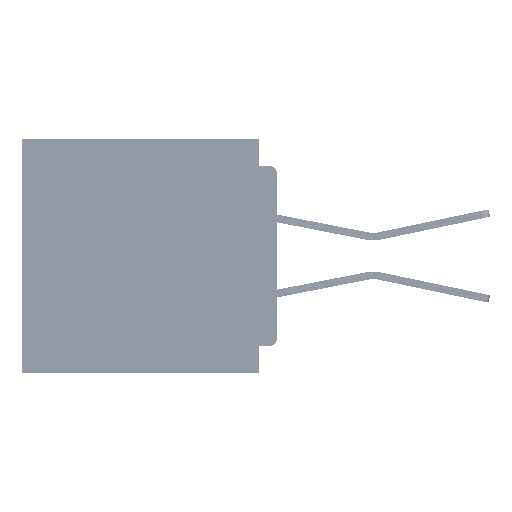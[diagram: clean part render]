
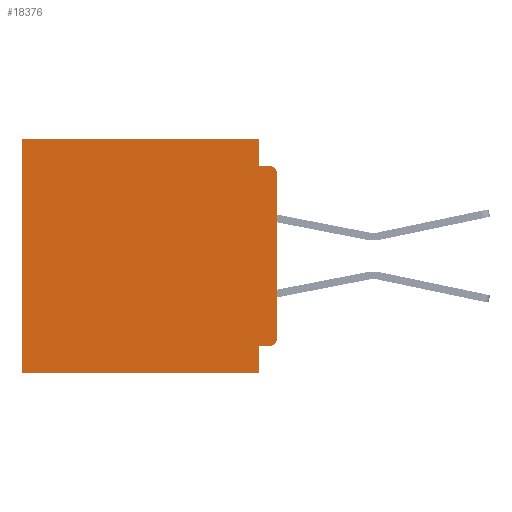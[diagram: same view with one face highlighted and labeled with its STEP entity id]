
A CAD part, left-side view. The second image highlights one B-rep face of the part: STEP entity #18376.
In plain terms, the highlighted planar face has unit normal (-1, 0, 0).
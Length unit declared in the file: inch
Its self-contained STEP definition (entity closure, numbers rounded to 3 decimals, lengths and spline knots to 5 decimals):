
#213 = CARTESIAN_POINT ( 'NONE',  ( 0.3, 0.437, -0.4 ) ) ;
#479 = ORIENTED_EDGE ( 'NONE', *, *, #10741, .F. ) ;
#855 = FACE_OUTER_BOUND ( 'NONE', #14915, .T. ) ;
#1376 = LINE ( 'NONE', #213, #41180 ) ;
#2153 = DIRECTION ( 'NONE',  ( 0., 0., -1. ) ) ;
#3269 = DIRECTION ( 'NONE',  ( 0., 1., 0. ) ) ;
#3931 = LINE ( 'NONE', #19192, #29967 ) ;
#5414 = DIRECTION ( 'NONE',  ( 0., 0., -1. ) ) ;
#5662 = CARTESIAN_POINT ( 'NONE',  ( 0.3, 0.031, -0.045 ) ) ;
#7006 = CARTESIAN_POINT ( 'NONE',  ( 0.3, 0.015, -0.34 ) ) ;
#7553 = VERTEX_POINT ( 'NONE', #53003 ) ;
#8582 = CARTESIAN_POINT ( 'NONE',  ( 0.3, 0., -0.045 ) ) ;
#9204 = LINE ( 'NONE', #8582, #48821 ) ;
#9430 = CARTESIAN_POINT ( 'NONE',  ( 0.3, 0.437, -0.4 ) ) ;
#9541 = VECTOR ( 'NONE', #35898, 39.37008 ) ;
#10218 = CARTESIAN_POINT ( 'NONE',  ( 0.3, 0., -0.4 ) ) ;
#10741 = EDGE_CURVE ( 'NONE', #64204, #25860, #42358, .T. ) ;
#12268 = EDGE_CURVE ( 'NONE', #49437, #56496, #38239, .T. ) ;
#12282 = EDGE_CURVE ( 'NONE', #60415, #41325, #48625, .T. ) ;
#12359 = DIRECTION ( 'NONE',  ( 0., 0., -1. ) ) ;
#13957 = DIRECTION ( 'NONE',  ( 0., -1., 0. ) ) ;
#14915 = EDGE_LOOP ( 'NONE', ( #58551, #46555, #37774, #23265, #29747, #54612, #479, #41886, #33028, #25817 ) ) ;
#17399 = VERTEX_POINT ( 'NONE', #35720 ) ;
#17871 = CARTESIAN_POINT ( 'NONE',  ( 0.3, 0.015, -0.06 ) ) ;
#18376 = ADVANCED_FACE ( 'NONE', ( #855 ), #38282, .F. ) ;
#19192 = CARTESIAN_POINT ( 'NONE',  ( 0.3, 0., 0. ) ) ;
#20373 = EDGE_CURVE ( 'NONE', #17399, #25860, #1376, .T. ) ;
#22192 = CARTESIAN_POINT ( 'NONE',  ( 0.3, 0.015, -0.355 ) ) ;
#22832 = DIRECTION ( 'NONE',  ( 0., 0., -1. ) ) ;
#23070 = DIRECTION ( 'NONE',  ( 0., 0., -1. ) ) ;
#23265 = ORIENTED_EDGE ( 'NONE', *, *, #12282, .F. ) ;
#23739 = EDGE_CURVE ( 'NONE', #28719, #64204, #46821, .T. ) ;
#24396 = DIRECTION ( 'NONE',  ( 0., 1., 0. ) ) ;
#25091 = LINE ( 'NONE', #10218, #9541 ) ;
#25817 = ORIENTED_EDGE ( 'NONE', *, *, #12268, .T. ) ;
#25860 = VERTEX_POINT ( 'NONE', #9430 ) ;
#27054 = VECTOR ( 'NONE', #3269, 39.37008 ) ;
#28719 = VERTEX_POINT ( 'NONE', #29001 ) ;
#29001 = CARTESIAN_POINT ( 'NONE',  ( 0.3, 0.031, -0.355 ) ) ;
#29029 = AXIS2_PLACEMENT_3D ( 'NONE', #63980, #33325, #2153 ) ;
#29156 = CARTESIAN_POINT ( 'NONE',  ( 0.3, 0., -0.355 ) ) ;
#29747 = ORIENTED_EDGE ( 'NONE', *, *, #48342, .T. ) ;
#29862 = EDGE_CURVE ( 'NONE', #41325, #7553, #9204, .T. ) ;
#29967 = VECTOR ( 'NONE', #24396, 39.37008 ) ;
#31392 = LINE ( 'NONE', #29156, #43482 ) ;
#33028 = ORIENTED_EDGE ( 'NONE', *, *, #49620, .F. ) ;
#33325 = DIRECTION ( 'NONE',  ( 1., 0., 0. ) ) ;
#34344 = DIRECTION ( 'NONE',  ( 0., 1., 0. ) ) ;
#35261 = AXIS2_PLACEMENT_3D ( 'NONE', #7006, #43345, #12359 ) ;
#35720 = CARTESIAN_POINT ( 'NONE',  ( 0.3, 0.437, 0. ) ) ;
#35807 = CARTESIAN_POINT ( 'NONE',  ( 0.3, 0.031, -0.4 ) ) ;
#35898 = DIRECTION ( 'NONE',  ( 0., 0., -1. ) ) ;
#37774 = ORIENTED_EDGE ( 'NONE', *, *, #29862, .F. ) ;
#38239 = CIRCLE ( 'NONE', #35261, 0.015 ) ;
#38282 = PLANE ( 'NONE',  #29029 ) ;
#38449 = EDGE_CURVE ( 'NONE', #64692, #56496, #25091, .T. ) ;
#41180 = VECTOR ( 'NONE', #5414, 39.37008 ) ;
#41325 = VERTEX_POINT ( 'NONE', #5662 ) ;
#41596 = CARTESIAN_POINT ( 'NONE',  ( 0.3, 0.031, 0. ) ) ;
#41886 = ORIENTED_EDGE ( 'NONE', *, *, #23739, .F. ) ;
#42358 = LINE ( 'NONE', #54743, #27054 ) ;
#43345 = DIRECTION ( 'NONE',  ( -1., 0., 0. ) ) ;
#43482 = VECTOR ( 'NONE', #34344, 39.37008 ) ;
#45660 = CARTESIAN_POINT ( 'NONE',  ( 0.3, 0., -0.34 ) ) ;
#46555 = ORIENTED_EDGE ( 'NONE', *, *, #49508, .T. ) ;
#46821 = LINE ( 'NONE', #35807, #50017 ) ;
#47587 = CARTESIAN_POINT ( 'NONE',  ( 0.3, 0., -0.06 ) ) ;
#48342 = EDGE_CURVE ( 'NONE', #60415, #17399, #3931, .T. ) ;
#48625 = LINE ( 'NONE', #58732, #62219 ) ;
#48821 = VECTOR ( 'NONE', #13957, 39.37008 ) ;
#49437 = VERTEX_POINT ( 'NONE', #22192 ) ;
#49508 = EDGE_CURVE ( 'NONE', #64692, #7553, #65037, .T. ) ;
#49620 = EDGE_CURVE ( 'NONE', #49437, #28719, #31392, .T. ) ;
#50017 = VECTOR ( 'NONE', #51013, 39.37008 ) ;
#51013 = DIRECTION ( 'NONE',  ( 0., 0., -1. ) ) ;
#53003 = CARTESIAN_POINT ( 'NONE',  ( 0.3, 0.015, -0.045 ) ) ;
#53452 = CARTESIAN_POINT ( 'NONE',  ( 0.3, 0.031, -0.4 ) ) ;
#53800 = DIRECTION ( 'NONE',  ( -1., 0., 0. ) ) ;
#54612 = ORIENTED_EDGE ( 'NONE', *, *, #20373, .T. ) ;
#54743 = CARTESIAN_POINT ( 'NONE',  ( 0.3, 0., -0.4 ) ) ;
#56496 = VERTEX_POINT ( 'NONE', #45660 ) ;
#58551 = ORIENTED_EDGE ( 'NONE', *, *, #38449, .F. ) ;
#58732 = CARTESIAN_POINT ( 'NONE',  ( 0.3, 0.031, 0. ) ) ;
#60415 = VERTEX_POINT ( 'NONE', #41596 ) ;
#62219 = VECTOR ( 'NONE', #22832, 39.37008 ) ;
#63980 = CARTESIAN_POINT ( 'NONE',  ( 0.3, 0., -0.4 ) ) ;
#64204 = VERTEX_POINT ( 'NONE', #53452 ) ;
#64548 = AXIS2_PLACEMENT_3D ( 'NONE', #17871, #53800, #23070 ) ;
#64692 = VERTEX_POINT ( 'NONE', #47587 ) ;
#65037 = CIRCLE ( 'NONE', #64548, 0.015 ) ;
